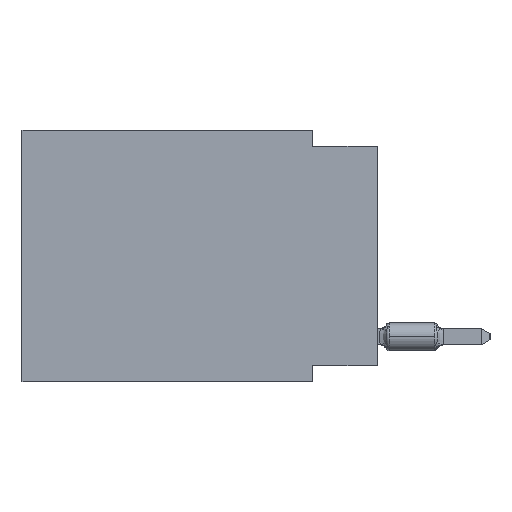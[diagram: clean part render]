
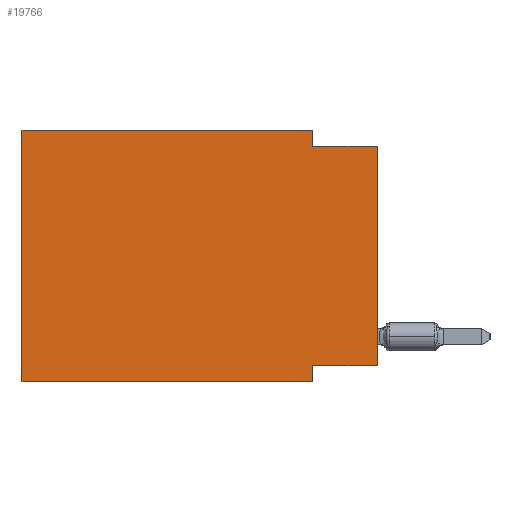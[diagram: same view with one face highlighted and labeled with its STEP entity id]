
A CAD part, left-side view. The second image highlights one B-rep face of the part: STEP entity #19766.
In plain terms, the highlighted planar face has unit normal (-1, 0, 0).
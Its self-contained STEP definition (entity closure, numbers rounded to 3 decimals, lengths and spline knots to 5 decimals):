
#1912 = CARTESIAN_POINT ( 'NONE',  ( 0., 0.1, 0. ) ) ;
#2309 = PLANE ( 'NONE',  #44896 ) ;
#4444 = EDGE_CURVE ( 'NONE', #62104, #10306, #34614, .T. ) ;
#4658 = VECTOR ( 'NONE', #51196, 39.37008 ) ;
#6534 = CARTESIAN_POINT ( 'NONE',  ( 0., 0., -0.365 ) ) ;
#7462 = CARTESIAN_POINT ( 'NONE',  ( 0., 0., 0. ) ) ;
#8281 = DIRECTION ( 'NONE',  ( 0., -1., 0. ) ) ;
#8925 = LINE ( 'NONE', #60768, #21108 ) ;
#9346 = DIRECTION ( 'NONE',  ( 0., -1., 0. ) ) ;
#10306 = VERTEX_POINT ( 'NONE', #59140 ) ;
#13541 = CARTESIAN_POINT ( 'NONE',  ( 0., 0.1, -0.025 ) ) ;
#15474 = DIRECTION ( 'NONE',  ( 1., 0., 0. ) ) ;
#16957 = VECTOR ( 'NONE', #65589, 39.37008 ) ;
#18881 = CARTESIAN_POINT ( 'NONE',  ( 0., 0.1, -0.39 ) ) ;
#19766 = ADVANCED_FACE ( 'NONE', ( #48172 ), #2309, .F. ) ;
#21108 = VECTOR ( 'NONE', #9346, 39.37008 ) ;
#21433 = LINE ( 'NONE', #7462, #81679 ) ;
#22191 = VERTEX_POINT ( 'NONE', #63102 ) ;
#24391 = LINE ( 'NONE', #36300, #71947 ) ;
#26242 = VECTOR ( 'NONE', #8281, 39.37008 ) ;
#32847 = EDGE_CURVE ( 'NONE', #65467, #62104, #24391, .T. ) ;
#34614 = LINE ( 'NONE', #40163, #26242 ) ;
#36300 = CARTESIAN_POINT ( 'NONE',  ( 0., 0.1, 0. ) ) ;
#39163 = EDGE_CURVE ( 'NONE', #71309, #39353, #71164, .T. ) ;
#39353 = VERTEX_POINT ( 'NONE', #47324 ) ;
#40163 = CARTESIAN_POINT ( 'NONE',  ( 0., 0., -0.025 ) ) ;
#40219 = EDGE_CURVE ( 'NONE', #61436, #71309, #78327, .T. ) ;
#40985 = CARTESIAN_POINT ( 'NONE',  ( 0., 0.55, 0. ) ) ;
#41093 = LINE ( 'NONE', #67016, #46128 ) ;
#42365 = ORIENTED_EDGE ( 'NONE', *, *, #4444, .F. ) ;
#42711 = ORIENTED_EDGE ( 'NONE', *, *, #67993, .T. ) ;
#44896 = AXIS2_PLACEMENT_3D ( 'NONE', #40985, #15474, #74103 ) ;
#46128 = VECTOR ( 'NONE', #67427, 39.37008 ) ;
#47022 = EDGE_CURVE ( 'NONE', #51192, #65467, #8925, .T. ) ;
#47324 = CARTESIAN_POINT ( 'NONE',  ( 0., 0.1, -0.39 ) ) ;
#47530 = VECTOR ( 'NONE', #56937, 39.37008 ) ;
#48172 = FACE_OUTER_BOUND ( 'NONE', #78040, .T. ) ;
#48778 = CARTESIAN_POINT ( 'NONE',  ( 0., 0.1, -0.365 ) ) ;
#49893 = DIRECTION ( 'NONE',  ( 0., 0., -1. ) ) ;
#51192 = VERTEX_POINT ( 'NONE', #72493 ) ;
#51196 = DIRECTION ( 'NONE',  ( 0., 0., -1. ) ) ;
#55990 = ORIENTED_EDGE ( 'NONE', *, *, #83300, .F. ) ;
#56123 = EDGE_CURVE ( 'NONE', #61436, #10306, #21433, .T. ) ;
#56937 = DIRECTION ( 'NONE',  ( 0., 0., 1. ) ) ;
#59140 = CARTESIAN_POINT ( 'NONE',  ( 0., 0., -0.025 ) ) ;
#60131 = DIRECTION ( 'NONE',  ( 0., 0., 1. ) ) ;
#60768 = CARTESIAN_POINT ( 'NONE',  ( 0., 0.55, 0. ) ) ;
#61436 = VERTEX_POINT ( 'NONE', #74020 ) ;
#62104 = VERTEX_POINT ( 'NONE', #13541 ) ;
#62271 = ORIENTED_EDGE ( 'NONE', *, *, #56123, .T. ) ;
#62899 = CARTESIAN_POINT ( 'NONE',  ( 0., 0.55, 0. ) ) ;
#63102 = CARTESIAN_POINT ( 'NONE',  ( 0., 0.55, -0.39 ) ) ;
#65230 = ORIENTED_EDGE ( 'NONE', *, *, #47022, .F. ) ;
#65467 = VERTEX_POINT ( 'NONE', #1912 ) ;
#65589 = DIRECTION ( 'NONE',  ( 0., 1., 0. ) ) ;
#65602 = ORIENTED_EDGE ( 'NONE', *, *, #32847, .F. ) ;
#67016 = CARTESIAN_POINT ( 'NONE',  ( 0., 0.55, -0.39 ) ) ;
#67427 = DIRECTION ( 'NONE',  ( 0., -1., 0. ) ) ;
#67993 = EDGE_CURVE ( 'NONE', #22191, #39353, #41093, .T. ) ;
#69284 = LINE ( 'NONE', #62899, #47530 ) ;
#69369 = ORIENTED_EDGE ( 'NONE', *, *, #39163, .F. ) ;
#70332 = ORIENTED_EDGE ( 'NONE', *, *, #40219, .F. ) ;
#71164 = LINE ( 'NONE', #18881, #4658 ) ;
#71309 = VERTEX_POINT ( 'NONE', #48778 ) ;
#71947 = VECTOR ( 'NONE', #49893, 39.37008 ) ;
#72493 = CARTESIAN_POINT ( 'NONE',  ( 0., 0.55, 0. ) ) ;
#74020 = CARTESIAN_POINT ( 'NONE',  ( 0., 0., -0.365 ) ) ;
#74103 = DIRECTION ( 'NONE',  ( 0., 0., -1. ) ) ;
#78040 = EDGE_LOOP ( 'NONE', ( #62271, #42365, #65602, #65230, #55990, #42711, #69369, #70332 ) ) ;
#78327 = LINE ( 'NONE', #6534, #16957 ) ;
#81679 = VECTOR ( 'NONE', #60131, 39.37008 ) ;
#83300 = EDGE_CURVE ( 'NONE', #22191, #51192, #69284, .T. ) ;
